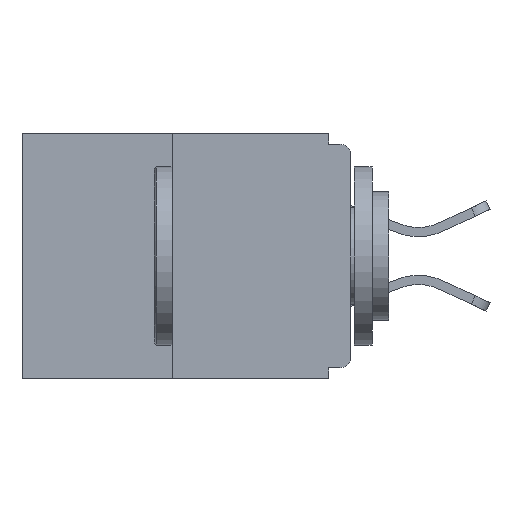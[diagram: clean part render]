
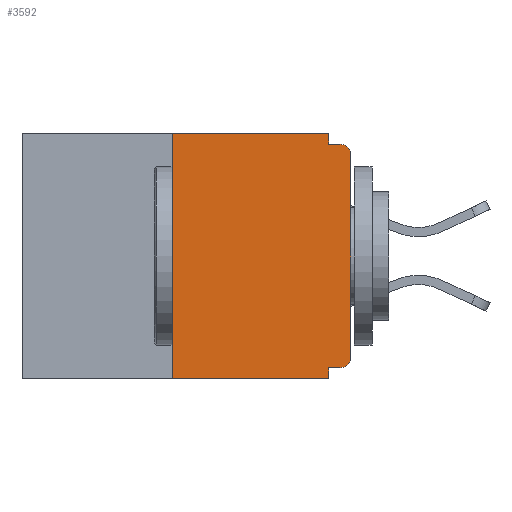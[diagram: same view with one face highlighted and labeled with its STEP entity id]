
A CAD part, left-side view. The second image highlights one B-rep face of the part: STEP entity #3592.
In plain terms, the highlighted planar face has unit normal (-1, 0, 0).
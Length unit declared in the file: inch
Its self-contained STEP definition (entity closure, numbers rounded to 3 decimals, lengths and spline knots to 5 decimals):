
#519 = DIRECTION ( 'NONE',  ( 0., 0., -1. ) ) ;
#567 = ORIENTED_EDGE ( 'NONE', *, *, #12674, .F. ) ;
#695 = ORIENTED_EDGE ( 'NONE', *, *, #21324, .T. ) ;
#2023 = VERTEX_POINT ( 'NONE', #21879 ) ;
#2201 = VERTEX_POINT ( 'NONE', #16453 ) ;
#2642 = VERTEX_POINT ( 'NONE', #17104 ) ;
#2720 = LINE ( 'NONE', #12936, #26510 ) ;
#3126 = DIRECTION ( 'NONE',  ( 0., 0., 1. ) ) ;
#3176 = ORIENTED_EDGE ( 'NONE', *, *, #26979, .F. ) ;
#3407 = DIRECTION ( 'NONE',  ( 0., 0., -1. ) ) ;
#3592 = ADVANCED_FACE ( 'NONE', ( #28239 ), #18020, .F. ) ;
#4494 = CARTESIAN_POINT ( 'NONE',  ( 0., 0.46, 0. ) ) ;
#4587 = DIRECTION ( 'NONE',  ( 0., -1., 0. ) ) ;
#5711 = DIRECTION ( 'NONE',  ( 0., 0., -1. ) ) ;
#5824 = EDGE_LOOP ( 'NONE', ( #25564, #6828, #21784, #15708, #13991, #12968, #13157, #695, #3176, #567 ) ) ;
#5876 = EDGE_CURVE ( 'NONE', #19953, #21175, #19581, .T. ) ;
#5983 = EDGE_CURVE ( 'NONE', #23848, #2642, #27475, .T. ) ;
#6307 = CIRCLE ( 'NONE', #6437, 0.015 ) ;
#6437 = AXIS2_PLACEMENT_3D ( 'NONE', #13141, #24402, #9085 ) ;
#6517 = CARTESIAN_POINT ( 'NONE',  ( 0., 0., -0.313 ) ) ;
#6611 = VECTOR ( 'NONE', #4587, 39.37008 ) ;
#6828 = ORIENTED_EDGE ( 'NONE', *, *, #13981, .F. ) ;
#7364 = VECTOR ( 'NONE', #17759, 39.37008 ) ;
#7919 = LINE ( 'NONE', #7974, #19325 ) ;
#7974 = CARTESIAN_POINT ( 'NONE',  ( 0., 0., 0. ) ) ;
#8256 = VERTEX_POINT ( 'NONE', #13386 ) ;
#8321 = DIRECTION ( 'NONE',  ( 0., -1., 0. ) ) ;
#8441 = CARTESIAN_POINT ( 'NONE',  ( 0., 0.015, -0.328 ) ) ;
#9085 = DIRECTION ( 'NONE',  ( 0., 0., -1. ) ) ;
#9211 = CARTESIAN_POINT ( 'NONE',  ( 0., 0.46, 0. ) ) ;
#9637 = LINE ( 'NONE', #22721, #10310 ) ;
#10310 = VECTOR ( 'NONE', #3126, 39.37008 ) ;
#11435 = DIRECTION ( 'NONE',  ( 0., 0., -1. ) ) ;
#11550 = EDGE_CURVE ( 'NONE', #19953, #23848, #13242, .T. ) ;
#11692 = VERTEX_POINT ( 'NONE', #18230 ) ;
#11724 = VERTEX_POINT ( 'NONE', #27101 ) ;
#12337 = CARTESIAN_POINT ( 'NONE',  ( 0., 0.031, -0.343 ) ) ;
#12674 = EDGE_CURVE ( 'NONE', #11724, #8256, #18693, .T. ) ;
#12684 = VECTOR ( 'NONE', #5711, 39.37008 ) ;
#12936 = CARTESIAN_POINT ( 'NONE',  ( 0., 0., -0.015 ) ) ;
#12968 = ORIENTED_EDGE ( 'NONE', *, *, #5876, .T. ) ;
#13141 = CARTESIAN_POINT ( 'NONE',  ( 0., 0.015, -0.03 ) ) ;
#13157 = ORIENTED_EDGE ( 'NONE', *, *, #13588, .T. ) ;
#13175 = LINE ( 'NONE', #4494, #6611 ) ;
#13242 = LINE ( 'NONE', #22180, #7364 ) ;
#13386 = CARTESIAN_POINT ( 'NONE',  ( 0., 0.031, -0.015 ) ) ;
#13588 = EDGE_CURVE ( 'NONE', #21175, #2201, #7919, .T. ) ;
#13981 = EDGE_CURVE ( 'NONE', #11692, #27426, #9637, .T. ) ;
#13991 = ORIENTED_EDGE ( 'NONE', *, *, #11550, .F. ) ;
#15164 = DIRECTION ( 'NONE',  ( 0., -1., 0. ) ) ;
#15708 = ORIENTED_EDGE ( 'NONE', *, *, #5983, .F. ) ;
#16453 = CARTESIAN_POINT ( 'NONE',  ( 0., 0., -0.03 ) ) ;
#16639 = CARTESIAN_POINT ( 'NONE',  ( 0., 0.031, 0. ) ) ;
#17104 = CARTESIAN_POINT ( 'NONE',  ( 0., 0.031, -0.343 ) ) ;
#17151 = VECTOR ( 'NONE', #15164, 39.37008 ) ;
#17759 = DIRECTION ( 'NONE',  ( 0., 1., 0. ) ) ;
#18020 = PLANE ( 'NONE',  #21280 ) ;
#18230 = CARTESIAN_POINT ( 'NONE',  ( 0., 0.25, -0.343 ) ) ;
#18693 = LINE ( 'NONE', #16639, #21443 ) ;
#19325 = VECTOR ( 'NONE', #23562, 39.37008 ) ;
#19581 = CIRCLE ( 'NONE', #20399, 0.015 ) ;
#19953 = VERTEX_POINT ( 'NONE', #8441 ) ;
#20399 = AXIS2_PLACEMENT_3D ( 'NONE', #22672, #24947, #519 ) ;
#20920 = LINE ( 'NONE', #21816, #17151 ) ;
#21175 = VERTEX_POINT ( 'NONE', #6517 ) ;
#21280 = AXIS2_PLACEMENT_3D ( 'NONE', #9211, #24615, #11435 ) ;
#21324 = EDGE_CURVE ( 'NONE', #2201, #2023, #6307, .T. ) ;
#21443 = VECTOR ( 'NONE', #3407, 39.37008 ) ;
#21784 = ORIENTED_EDGE ( 'NONE', *, *, #22241, .T. ) ;
#21786 = CARTESIAN_POINT ( 'NONE',  ( 0., 0.031, -0.328 ) ) ;
#21816 = CARTESIAN_POINT ( 'NONE',  ( 0., 0.46, -0.343 ) ) ;
#21879 = CARTESIAN_POINT ( 'NONE',  ( 0., 0.015, -0.015 ) ) ;
#22180 = CARTESIAN_POINT ( 'NONE',  ( 0., 0., -0.328 ) ) ;
#22241 = EDGE_CURVE ( 'NONE', #11692, #2642, #20920, .T. ) ;
#22672 = CARTESIAN_POINT ( 'NONE',  ( 0., 0.015, -0.313 ) ) ;
#22721 = CARTESIAN_POINT ( 'NONE',  ( 0., 0.25, 0. ) ) ;
#23294 = CARTESIAN_POINT ( 'NONE',  ( 0., 0.25, 0. ) ) ;
#23562 = DIRECTION ( 'NONE',  ( 0., 0., 1. ) ) ;
#23848 = VERTEX_POINT ( 'NONE', #21786 ) ;
#24402 = DIRECTION ( 'NONE',  ( -1., 0., 0. ) ) ;
#24615 = DIRECTION ( 'NONE',  ( 1., 0., 0. ) ) ;
#24947 = DIRECTION ( 'NONE',  ( -1., 0., 0. ) ) ;
#25564 = ORIENTED_EDGE ( 'NONE', *, *, #28177, .F. ) ;
#26510 = VECTOR ( 'NONE', #8321, 39.37008 ) ;
#26979 = EDGE_CURVE ( 'NONE', #8256, #2023, #2720, .T. ) ;
#27101 = CARTESIAN_POINT ( 'NONE',  ( 0., 0.031, 0. ) ) ;
#27426 = VERTEX_POINT ( 'NONE', #23294 ) ;
#27475 = LINE ( 'NONE', #12337, #12684 ) ;
#28177 = EDGE_CURVE ( 'NONE', #27426, #11724, #13175, .T. ) ;
#28239 = FACE_OUTER_BOUND ( 'NONE', #5824, .T. ) ;
